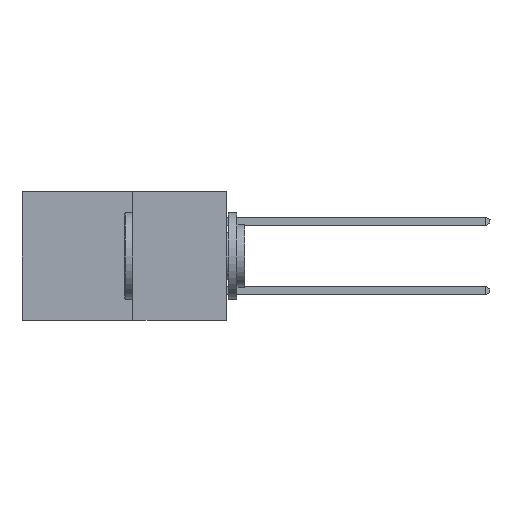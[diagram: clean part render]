
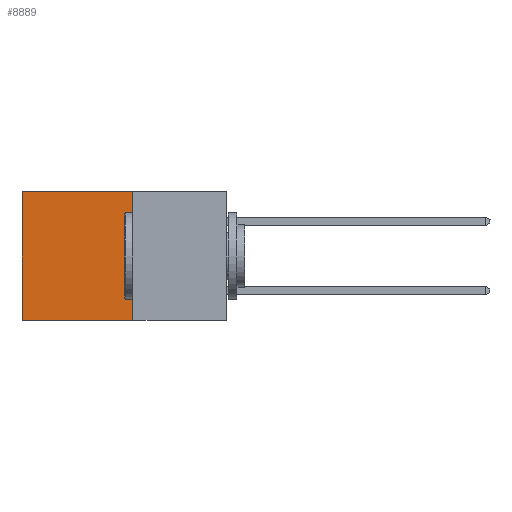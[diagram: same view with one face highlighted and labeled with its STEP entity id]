
A CAD part, left-side view. The second image highlights one B-rep face of the part: STEP entity #8889.
In plain terms, the highlighted planar face has unit normal (-1, 0, 0).
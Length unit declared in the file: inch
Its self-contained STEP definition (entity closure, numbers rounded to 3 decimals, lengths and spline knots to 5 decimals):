
#460 = EDGE_CURVE ( 'NONE', #8230, #14815, #1803, .T. ) ;
#916 = CARTESIAN_POINT ( 'NONE',  ( 0.277, 0.59, 0. ) ) ;
#986 = CARTESIAN_POINT ( 'NONE',  ( 0.277, 0.27, 0. ) ) ;
#1803 = LINE ( 'NONE', #9984, #21908 ) ;
#2431 = VECTOR ( 'NONE', #2983, 39.37008 ) ;
#2983 = DIRECTION ( 'NONE',  ( 0., 1., 0. ) ) ;
#4157 = DIRECTION ( 'NONE',  ( 0., 0., -1. ) ) ;
#6446 = FACE_OUTER_BOUND ( 'NONE', #16347, .T. ) ;
#6786 = PLANE ( 'NONE',  #20887 ) ;
#6888 = DIRECTION ( 'NONE',  ( 1., 0., 0. ) ) ;
#6999 = CARTESIAN_POINT ( 'NONE',  ( 0.277, 0.59, -0.37 ) ) ;
#7298 = ORIENTED_EDGE ( 'NONE', *, *, #20919, .F. ) ;
#8098 = ORIENTED_EDGE ( 'NONE', *, *, #24842, .T. ) ;
#8230 = VERTEX_POINT ( 'NONE', #986 ) ;
#8889 = ADVANCED_FACE ( 'NONE', ( #6446 ), #6786, .F. ) ;
#9984 = CARTESIAN_POINT ( 'NONE',  ( 0.277, 0.27, -0.37 ) ) ;
#12428 = EDGE_CURVE ( 'NONE', #18562, #13737, #14279, .T. ) ;
#13098 = ORIENTED_EDGE ( 'NONE', *, *, #12428, .T. ) ;
#13737 = VERTEX_POINT ( 'NONE', #6999 ) ;
#14262 = CARTESIAN_POINT ( 'NONE',  ( 0.277, 0.59, -0.37 ) ) ;
#14279 = LINE ( 'NONE', #14262, #18906 ) ;
#14815 = VERTEX_POINT ( 'NONE', #16662 ) ;
#15052 = CARTESIAN_POINT ( 'NONE',  ( 0.277, 0.27, 0. ) ) ;
#16347 = EDGE_LOOP ( 'NONE', ( #13098, #7298, #22676, #8098 ) ) ;
#16662 = CARTESIAN_POINT ( 'NONE',  ( 0.277, 0.27, -0.37 ) ) ;
#17039 = DIRECTION ( 'NONE',  ( 0., 1., 0. ) ) ;
#17089 = CARTESIAN_POINT ( 'NONE',  ( 0.277, 0.27, -0.37 ) ) ;
#17888 = LINE ( 'NONE', #17089, #2431 ) ;
#18562 = VERTEX_POINT ( 'NONE', #916 ) ;
#18898 = CARTESIAN_POINT ( 'NONE',  ( 0.277, 0.27, -0.37 ) ) ;
#18906 = VECTOR ( 'NONE', #4157, 39.37008 ) ;
#20383 = DIRECTION ( 'NONE',  ( 0., 0., -1. ) ) ;
#20887 = AXIS2_PLACEMENT_3D ( 'NONE', #18898, #6888, #20892 ) ;
#20892 = DIRECTION ( 'NONE',  ( 0., 0., -1. ) ) ;
#20919 = EDGE_CURVE ( 'NONE', #14815, #13737, #17888, .T. ) ;
#21908 = VECTOR ( 'NONE', #20383, 39.37008 ) ;
#22676 = ORIENTED_EDGE ( 'NONE', *, *, #460, .F. ) ;
#23613 = VECTOR ( 'NONE', #17039, 39.37008 ) ;
#24248 = LINE ( 'NONE', #15052, #23613 ) ;
#24842 = EDGE_CURVE ( 'NONE', #8230, #18562, #24248, .T. ) ;
